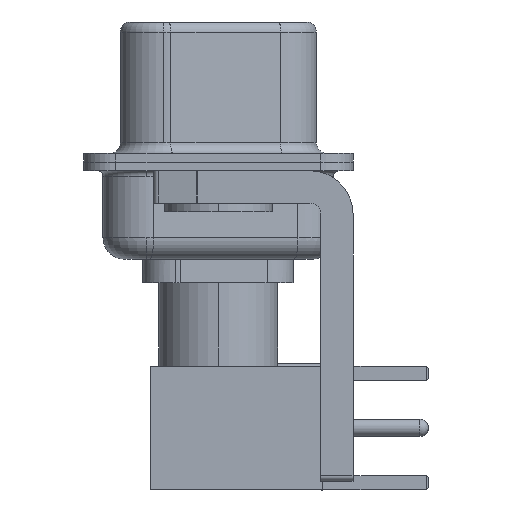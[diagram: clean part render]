
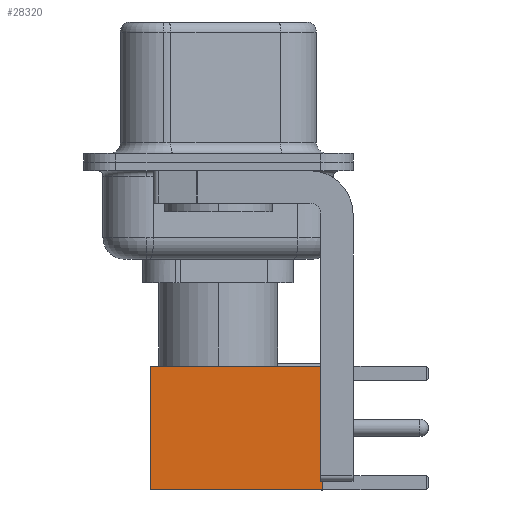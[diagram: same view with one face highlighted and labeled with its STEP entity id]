
A CAD part, left-side view. The second image highlights one B-rep face of the part: STEP entity #28320.
In plain terms, the highlighted face is planar.
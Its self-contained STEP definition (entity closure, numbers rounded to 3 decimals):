
#1019 = ORIENTED_EDGE ( 'NONE', *, *, #21310, .T. ) ;
#2107 = EDGE_CURVE ( 'NONE', #17556, #28584, #13134, .T. ) ;
#2596 = CARTESIAN_POINT ( 'NONE',  ( -2.875, 2.875, 0. ) ) ;
#3185 = VECTOR ( 'NONE', #29030, 1000. ) ;
#3721 = ORIENTED_EDGE ( 'NONE', *, *, #17840, .F. ) ;
#4644 = ORIENTED_EDGE ( 'NONE', *, *, #20610, .F. ) ;
#4724 = PLANE ( 'NONE',  #15487 ) ;
#4815 = ORIENTED_EDGE ( 'NONE', *, *, #2107, .T. ) ;
#6112 = LINE ( 'NONE', #30157, #29630 ) ;
#6479 = VERTEX_POINT ( 'NONE', #17697 ) ;
#7620 = EDGE_LOOP ( 'NONE', ( #4815, #1019, #4644, #3721 ) ) ;
#8779 = VECTOR ( 'NONE', #19994, 1000. ) ;
#10414 = LINE ( 'NONE', #15710, #28475 ) ;
#10855 = VERTEX_POINT ( 'NONE', #12167 ) ;
#12167 = CARTESIAN_POINT ( 'NONE',  ( -2.875, 2.875, 0. ) ) ;
#12870 = DIRECTION ( 'NONE',  ( -1., 0., 0. ) ) ;
#13134 = LINE ( 'NONE', #27531, #8779 ) ;
#13388 = CARTESIAN_POINT ( 'NONE',  ( 2.875, 2.875, 0. ) ) ;
#14056 = DIRECTION ( 'NONE',  ( 0., 0., 1. ) ) ;
#15487 = AXIS2_PLACEMENT_3D ( 'NONE', #31175, #19305, #14056 ) ;
#15677 = CARTESIAN_POINT ( 'NONE',  ( 2.875, 2.875, 8. ) ) ;
#15710 = CARTESIAN_POINT ( 'NONE',  ( 0., 2.875, 0. ) ) ;
#17500 = LINE ( 'NONE', #2596, #3185 ) ;
#17556 = VERTEX_POINT ( 'NONE', #15677 ) ;
#17697 = CARTESIAN_POINT ( 'NONE',  ( -2.875, 2.875, 8. ) ) ;
#17840 = EDGE_CURVE ( 'NONE', #17556, #6479, #6112, .T. ) ;
#19305 = DIRECTION ( 'NONE',  ( 0., 1., 0. ) ) ;
#19994 = DIRECTION ( 'NONE',  ( 0., 0., -1. ) ) ;
#20166 = DIRECTION ( 'NONE',  ( -1., 0., 0. ) ) ;
#20610 = EDGE_CURVE ( 'NONE', #6479, #10855, #17500, .T. ) ;
#21310 = EDGE_CURVE ( 'NONE', #28584, #10855, #10414, .T. ) ;
#27531 = CARTESIAN_POINT ( 'NONE',  ( 2.875, 2.875, 0. ) ) ;
#28320 = ADVANCED_FACE ( 'NONE', ( #31478 ), #4724, .T. ) ;
#28475 = VECTOR ( 'NONE', #20166, 1000. ) ;
#28584 = VERTEX_POINT ( 'NONE', #13388 ) ;
#29030 = DIRECTION ( 'NONE',  ( 0., 0., -1. ) ) ;
#29630 = VECTOR ( 'NONE', #12870, 1000. ) ;
#30157 = CARTESIAN_POINT ( 'NONE',  ( 0., 2.875, 8. ) ) ;
#31175 = CARTESIAN_POINT ( 'NONE',  ( 2.875, 2.875, 0. ) ) ;
#31478 = FACE_OUTER_BOUND ( 'NONE', #7620, .T. ) ;
